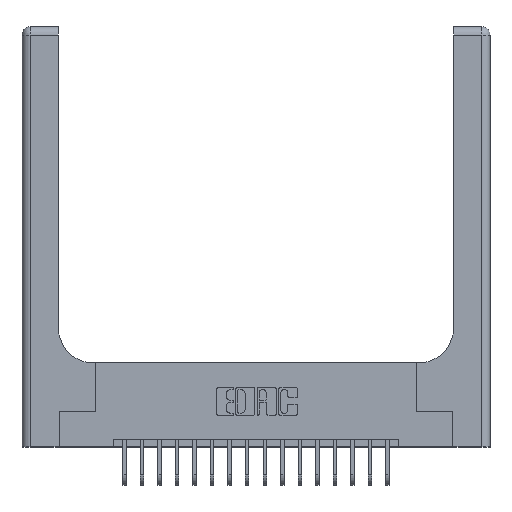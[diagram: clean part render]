
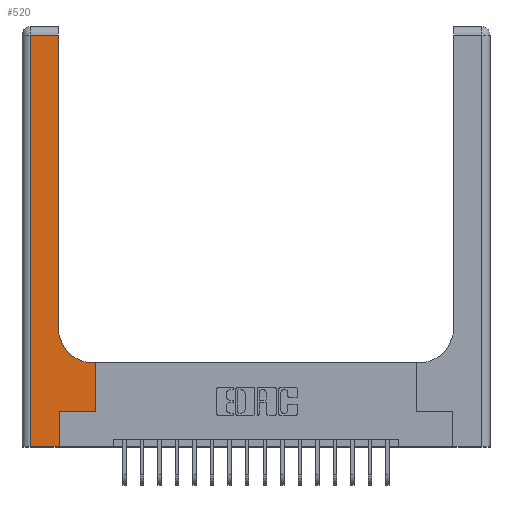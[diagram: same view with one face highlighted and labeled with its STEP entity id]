
A CAD part, top view. The second image highlights one B-rep face of the part: STEP entity #520.
In plain terms, the highlighted planar face has unit normal (0, 0, 1).
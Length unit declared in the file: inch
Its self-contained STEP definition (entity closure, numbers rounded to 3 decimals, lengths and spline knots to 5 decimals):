
#179 = EDGE_CURVE ( 'NONE', #4726, #8597, #16341, .T. ) ;
#434 = ORIENTED_EDGE ( 'NONE', *, *, #179, .T. ) ;
#520 = ADVANCED_FACE ( 'NONE', ( #15661 ), #8553, .F. ) ;
#530 = EDGE_CURVE ( 'NONE', #8070, #10522, #12749, .T. ) ;
#561 = AXIS2_PLACEMENT_3D ( 'NONE', #16300, #7689, #17689 ) ;
#571 = VERTEX_POINT ( 'NONE', #12613 ) ;
#678 = ORIENTED_EDGE ( 'NONE', *, *, #12961, .T. ) ;
#840 = VECTOR ( 'NONE', #16311, 39.37008 ) ;
#1299 = LINE ( 'NONE', #6255, #840 ) ;
#1379 = CARTESIAN_POINT ( 'NONE',  ( 0.26, 2.94, 0.37 ) ) ;
#1950 = CARTESIAN_POINT ( 'NONE',  ( 0.26, 0.85, 0.37 ) ) ;
#1954 = VECTOR ( 'NONE', #3774, 39.37008 ) ;
#2083 = DIRECTION ( 'NONE',  ( 0., 1., 0. ) ) ;
#2461 = CARTESIAN_POINT ( 'NONE',  ( 0.265, 0.25, 0.37 ) ) ;
#2859 = VERTEX_POINT ( 'NONE', #1950 ) ;
#3774 = DIRECTION ( 'NONE',  ( 0., 1., 0. ) ) ;
#3911 = ORIENTED_EDGE ( 'NONE', *, *, #530, .T. ) ;
#3926 = CARTESIAN_POINT ( 'NONE',  ( 0.528, 0.25, 0.37 ) ) ;
#4129 = VECTOR ( 'NONE', #2083, 39.37008 ) ;
#4726 = VERTEX_POINT ( 'NONE', #14505 ) ;
#4840 = CARTESIAN_POINT ( 'NONE',  ( 0.265, 0., 0.37 ) ) ;
#4896 = EDGE_LOOP ( 'NONE', ( #11188, #678, #14761, #434, #5213, #17371, #3911, #5189, #15051 ) ) ;
#5189 = ORIENTED_EDGE ( 'NONE', *, *, #12378, .T. ) ;
#5213 = ORIENTED_EDGE ( 'NONE', *, *, #12250, .T. ) ;
#5843 = DIRECTION ( 'NONE',  ( 0., -1., 0. ) ) ;
#5919 = LINE ( 'NONE', #7951, #13146 ) ;
#5996 = DIRECTION ( 'NONE',  ( -1., 0., 0. ) ) ;
#6100 = DIRECTION ( 'NONE',  ( 0., 0., -1. ) ) ;
#6255 = CARTESIAN_POINT ( 'NONE',  ( 0.265, 0., 0.37 ) ) ;
#6555 = CARTESIAN_POINT ( 'NONE',  ( 0., 3., 0.37 ) ) ;
#6597 = VECTOR ( 'NONE', #15454, 39.37008 ) ;
#7182 = EDGE_CURVE ( 'NONE', #12773, #2859, #16277, .T. ) ;
#7689 = DIRECTION ( 'NONE',  ( 0., 0., -1. ) ) ;
#7762 = EDGE_CURVE ( 'NONE', #2859, #18686, #13567, .T. ) ;
#7951 = CARTESIAN_POINT ( 'NONE',  ( 0.26, 0.6, 0.37 ) ) ;
#8070 = VERTEX_POINT ( 'NONE', #10390 ) ;
#8300 = CARTESIAN_POINT ( 'NONE',  ( 0.265, 0.25, 0.37 ) ) ;
#8553 = PLANE ( 'NONE',  #10173 ) ;
#8597 = VERTEX_POINT ( 'NONE', #4840 ) ;
#8718 = VECTOR ( 'NONE', #9931, 39.37008 ) ;
#9124 = EDGE_CURVE ( 'NONE', #571, #4726, #17097, .T. ) ;
#9416 = DIRECTION ( 'NONE',  ( -1., 0., 0. ) ) ;
#9505 = VERTEX_POINT ( 'NONE', #2461 ) ;
#9576 = CARTESIAN_POINT ( 'NONE',  ( 0.26, 3., 0.37 ) ) ;
#9762 = DIRECTION ( 'NONE',  ( 1., 0., 0. ) ) ;
#9823 = CARTESIAN_POINT ( 'NONE',  ( 0., 0., 0.37 ) ) ;
#9931 = DIRECTION ( 'NONE',  ( 1., 0., 0. ) ) ;
#10173 = AXIS2_PLACEMENT_3D ( 'NONE', #6555, #6100, #5996 ) ;
#10390 = CARTESIAN_POINT ( 'NONE',  ( 0.528, 0.25, 0.37 ) ) ;
#10434 = VECTOR ( 'NONE', #9762, 39.37008 ) ;
#10522 = VERTEX_POINT ( 'NONE', #17575 ) ;
#11188 = ORIENTED_EDGE ( 'NONE', *, *, #7762, .T. ) ;
#12250 = EDGE_CURVE ( 'NONE', #8597, #9505, #1299, .T. ) ;
#12378 = EDGE_CURVE ( 'NONE', #10522, #12773, #5919, .T. ) ;
#12613 = CARTESIAN_POINT ( 'NONE',  ( 0.06, 2.94, 0.37 ) ) ;
#12749 = LINE ( 'NONE', #3926, #4129 ) ;
#12773 = VERTEX_POINT ( 'NONE', #17922 ) ;
#12961 = EDGE_CURVE ( 'NONE', #18686, #571, #14689, .T. ) ;
#12984 = EDGE_CURVE ( 'NONE', #9505, #8070, #18005, .T. ) ;
#13146 = VECTOR ( 'NONE', #9416, 39.37008 ) ;
#13317 = VECTOR ( 'NONE', #5843, 39.37008 ) ;
#13567 = LINE ( 'NONE', #9576, #1954 ) ;
#14021 = CARTESIAN_POINT ( 'NONE',  ( 0., 2.94, 0.37 ) ) ;
#14505 = CARTESIAN_POINT ( 'NONE',  ( 0.06, 0., 0.37 ) ) ;
#14689 = LINE ( 'NONE', #14021, #6597 ) ;
#14761 = ORIENTED_EDGE ( 'NONE', *, *, #9124, .T. ) ;
#15051 = ORIENTED_EDGE ( 'NONE', *, *, #7182, .T. ) ;
#15454 = DIRECTION ( 'NONE',  ( -1., 0., 0. ) ) ;
#15661 = FACE_OUTER_BOUND ( 'NONE', #4896, .T. ) ;
#15933 = CARTESIAN_POINT ( 'NONE',  ( 0.06, 3., 0.37 ) ) ;
#16277 = CIRCLE ( 'NONE', #561, 0.25 ) ;
#16300 = CARTESIAN_POINT ( 'NONE',  ( 0.51, 0.85, 0.37 ) ) ;
#16311 = DIRECTION ( 'NONE',  ( 0., 1., 0. ) ) ;
#16341 = LINE ( 'NONE', #9823, #8718 ) ;
#17097 = LINE ( 'NONE', #15933, #13317 ) ;
#17371 = ORIENTED_EDGE ( 'NONE', *, *, #12984, .T. ) ;
#17575 = CARTESIAN_POINT ( 'NONE',  ( 0.528, 0.6, 0.37 ) ) ;
#17689 = DIRECTION ( 'NONE',  ( 1., 0., 0. ) ) ;
#17922 = CARTESIAN_POINT ( 'NONE',  ( 0.51, 0.6, 0.37 ) ) ;
#18005 = LINE ( 'NONE', #8300, #10434 ) ;
#18686 = VERTEX_POINT ( 'NONE', #1379 ) ;
